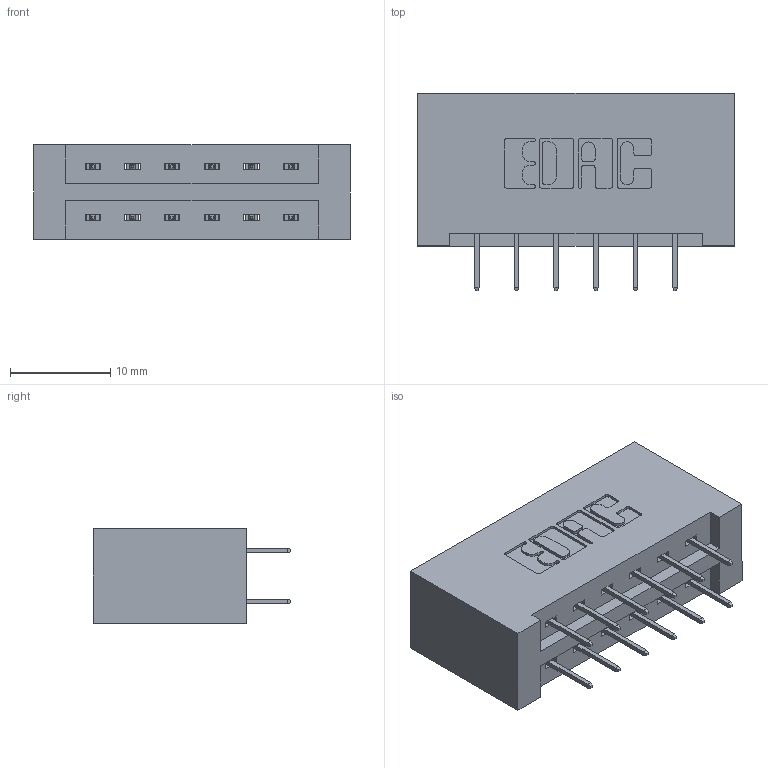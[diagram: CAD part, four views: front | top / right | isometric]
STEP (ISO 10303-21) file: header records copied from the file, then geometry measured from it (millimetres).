
FILE_DESCRIPTION (( 'STEP AP203' ), '1' );
FILE_NAME ('387-012-524-201.STEP', '2019-10-15T19:38:45', ( '' ), ( '' ), 'SwSTEP 2.0', 'SolidWorks 2016', '' );
FILE_SCHEMA (( 'CONFIG_CONTROL_DESIGN' ));
Length unit declared in the file: inch
Products named in the file (3): 337 Part_No Mounting Lugs; 387-012-524-201; 345-292-001_345-293-124
Assembly tree (13 placements, depth 2):
  387-012-524-201
    337 Part_No Mounting Lugs
    345-292-001_345-293-124  x12
Bounding box: 31.65 x 19.69 x 9.4 mm (x, y, z)
Volume: 3598.7 mm3; surface area: 3718.5 mm2
Topology: 13 solids, 13 shells, 802 faces, 2267 edges, 1462 vertices
Faces by surface type: plane 594, cylinder 208
Entity records: 9105 total; most frequent: CARTESIAN_POINT 1562, ORIENTED_EDGE 1498, DIRECTION 1389, EDGE_CURVE 749, LINE 633, VECTOR 633, VERTEX_POINT 494, AXIS2_PLACEMENT_3D 378
